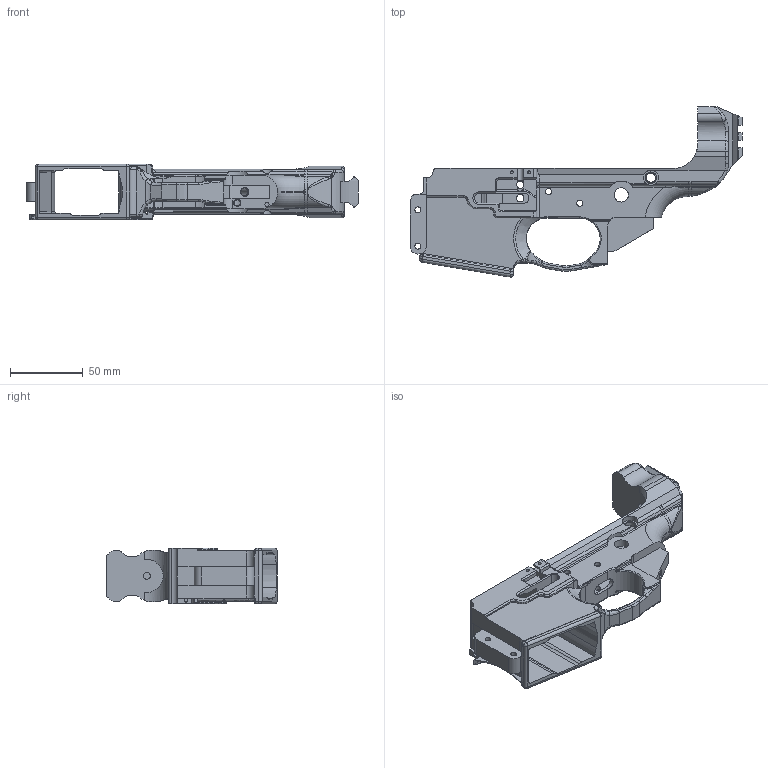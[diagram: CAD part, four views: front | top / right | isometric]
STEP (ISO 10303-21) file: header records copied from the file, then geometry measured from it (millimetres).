
FILE_DESCRIPTION(/* description */ (''),/* implementation_level */ '2;1');
FILE_NAME(/* name */ 'MEPR-X.step',/* time_stamp */ '2022-12-27T02:33:57-05:00',/* author */ (''),/* organization */ (''),/* preprocessor_version */ 'ST-DEVELOPER v19.2',/* originating_system */ 'Autodesk Translation Framework v11.17.0.187',/* authorisation */ '');
FILE_SCHEMA (('AUTOMOTIVE_DESIGN { 1 0 10303 214 3 1 1 }'));
Length unit declared in the file: millimetre
Products named in the file (1): MPX BODY
Bounding box: 228.28 x 117.02 x 38.45 mm (x, y, z)
Volume: 170126.9 mm3; surface area: 64378.7 mm2
Topology: 1 solids, 1 shells, 655 faces, 1755 edges, 1088 vertices
Faces by surface type: cylinder 247, plane 219, bspline 94, torus 65, cone 15, sphere 15
Full cylindrical faces by diameter (mm): 1.75 x2, 2 x4, 2.5 x1, 2.85 x1, 4 x2, 4.2 x1, 4.262 x4, 4.75 x1, 4.9 x1, 5 x1, 5.15 x1, 5.537 x1, 6.35 x2, 7.026 x1, 7.8 x1, 9.85 x2, 10.476 x2
Entity records: 28245 total; most frequent: CARTESIAN_POINT 12134, ORIENTED_EDGE 3492, DIRECTION 3284, EDGE_CURVE 1746, AXIS2_PLACEMENT_3D 1249, VERTEX_POINT 1088, LINE 786, VECTOR 786
